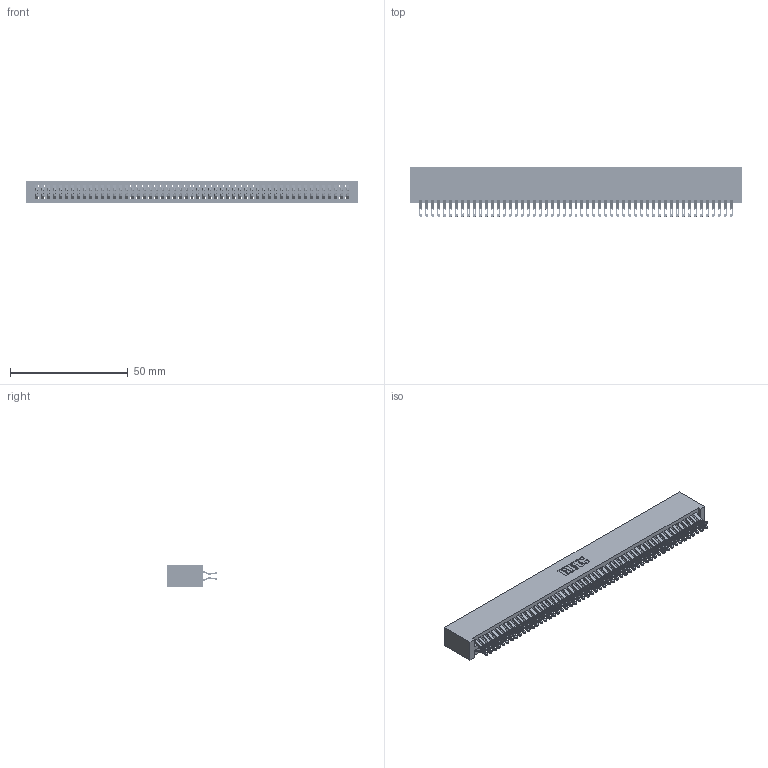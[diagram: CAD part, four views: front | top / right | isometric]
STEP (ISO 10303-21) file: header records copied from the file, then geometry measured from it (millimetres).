
FILE_DESCRIPTION (( 'STEP AP203' ), '1' );
FILE_NAME ('345-106-555-201.STEP', '2018-10-07T03:15:50', ( '' ), ( '' ), 'SwSTEP 2.0', 'SolidWorks 2016', '' );
FILE_SCHEMA (( 'CONFIG_CONTROL_DESIGN' ));
Length unit declared in the file: inch
Products named in the file (3): 345-292-001_555 Tail; 345-106-555-201; 345 Part_No Mounting Lugs
Assembly tree (107 placements, depth 2):
  345-106-555-201
    345 Part_No Mounting Lugs
    345-292-001_555 Tail  x106
Bounding box: 141.22 x 21.13 x 9.4 mm (x, y, z)
Volume: 14744.1 mm3; surface area: 23380 mm2
Topology: 107 solids, 107 shells, 6054 faces, 19079 edges, 12718 vertices
Faces by surface type: plane 3362, cylinder 2692
Entity records: 40153 total; most frequent: CARTESIAN_POINT 6754, ORIENTED_EDGE 6658, DIRECTION 5905, EDGE_CURVE 3329, LINE 2973, VECTOR 2973, VERTEX_POINT 2218, AXIS2_PLACEMENT_3D 1466
